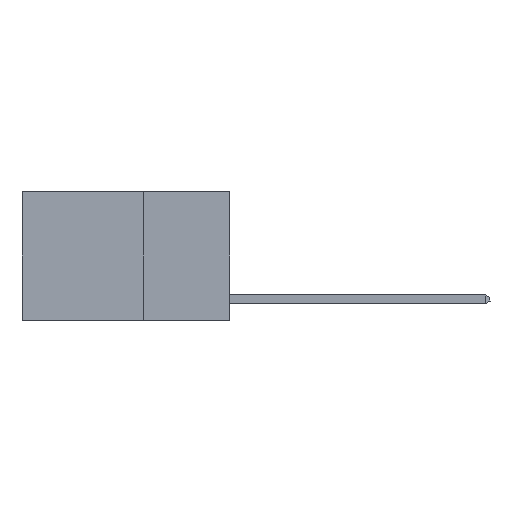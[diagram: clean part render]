
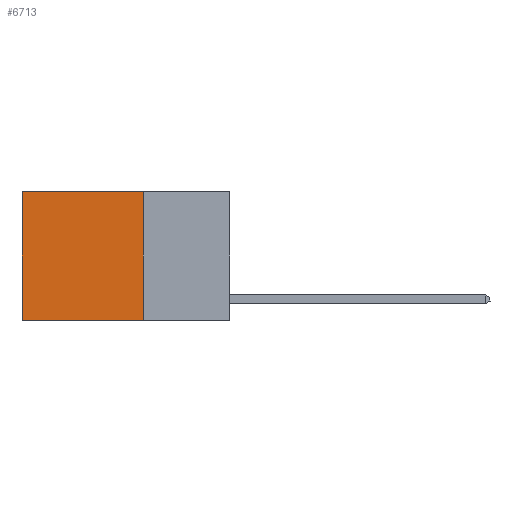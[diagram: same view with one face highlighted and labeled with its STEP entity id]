
A CAD part, left-side view. The second image highlights one B-rep face of the part: STEP entity #6713.
In plain terms, the highlighted planar face has unit normal (-1, 0, 0).
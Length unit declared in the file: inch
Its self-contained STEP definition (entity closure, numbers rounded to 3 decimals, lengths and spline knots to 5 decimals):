
#35 = AXIS2_PLACEMENT_3D ( 'NONE', #5629, #7611, #21442 ) ;
#451 = ORIENTED_EDGE ( 'NONE', *, *, #20700, .F. ) ;
#491 = CARTESIAN_POINT ( 'NONE',  ( 0.2625, 0.6, -0.37 ) ) ;
#2511 = CARTESIAN_POINT ( 'NONE',  ( 0.2625, 0.25, 0. ) ) ;
#2878 = EDGE_CURVE ( 'NONE', #9598, #17815, #17675, .T. ) ;
#4492 = DIRECTION ( 'NONE',  ( 0., 0., -1. ) ) ;
#5245 = CARTESIAN_POINT ( 'NONE',  ( 0.2625, 0.25, -0.37 ) ) ;
#5629 = CARTESIAN_POINT ( 'NONE',  ( 0.2625, 0.25, 0. ) ) ;
#6182 = VECTOR ( 'NONE', #8180, 39.37008 ) ;
#6309 = EDGE_LOOP ( 'NONE', ( #20981, #13425, #451, #21154 ) ) ;
#6713 = ADVANCED_FACE ( 'NONE', ( #12693 ), #17408, .F. ) ;
#6799 = LINE ( 'NONE', #14038, #6182 ) ;
#7611 = DIRECTION ( 'NONE',  ( 1., 0., 0. ) ) ;
#8180 = DIRECTION ( 'NONE',  ( 0., 1., 0. ) ) ;
#9582 = CARTESIAN_POINT ( 'NONE',  ( 0.2625, 0.6, 0. ) ) ;
#9598 = VERTEX_POINT ( 'NONE', #12899 ) ;
#10004 = LINE ( 'NONE', #16629, #24545 ) ;
#10158 = EDGE_CURVE ( 'NONE', #11591, #17815, #10004, .T. ) ;
#10416 = CARTESIAN_POINT ( 'NONE',  ( 0.2625, 0.25, 0. ) ) ;
#11591 = VERTEX_POINT ( 'NONE', #5245 ) ;
#12473 = VECTOR ( 'NONE', #13563, 39.37008 ) ;
#12693 = FACE_OUTER_BOUND ( 'NONE', #6309, .T. ) ;
#12899 = CARTESIAN_POINT ( 'NONE',  ( 0.2625, 0.6, 0. ) ) ;
#13425 = ORIENTED_EDGE ( 'NONE', *, *, #10158, .F. ) ;
#13563 = DIRECTION ( 'NONE',  ( 0., 0., -1. ) ) ;
#14038 = CARTESIAN_POINT ( 'NONE',  ( 0.2625, 0.25, 0. ) ) ;
#15144 = VECTOR ( 'NONE', #4492, 39.37008 ) ;
#16629 = CARTESIAN_POINT ( 'NONE',  ( 0.2625, 0.25, -0.37 ) ) ;
#17408 = PLANE ( 'NONE',  #35 ) ;
#17675 = LINE ( 'NONE', #9582, #12473 ) ;
#17815 = VERTEX_POINT ( 'NONE', #491 ) ;
#20700 = EDGE_CURVE ( 'NONE', #24122, #11591, #25058, .T. ) ;
#20981 = ORIENTED_EDGE ( 'NONE', *, *, #2878, .T. ) ;
#21154 = ORIENTED_EDGE ( 'NONE', *, *, #21232, .T. ) ;
#21232 = EDGE_CURVE ( 'NONE', #24122, #9598, #6799, .T. ) ;
#21442 = DIRECTION ( 'NONE',  ( 0., 0., -1. ) ) ;
#24122 = VERTEX_POINT ( 'NONE', #10416 ) ;
#24545 = VECTOR ( 'NONE', #24610, 39.37008 ) ;
#24610 = DIRECTION ( 'NONE',  ( 0., 1., 0. ) ) ;
#25058 = LINE ( 'NONE', #2511, #15144 ) ;
